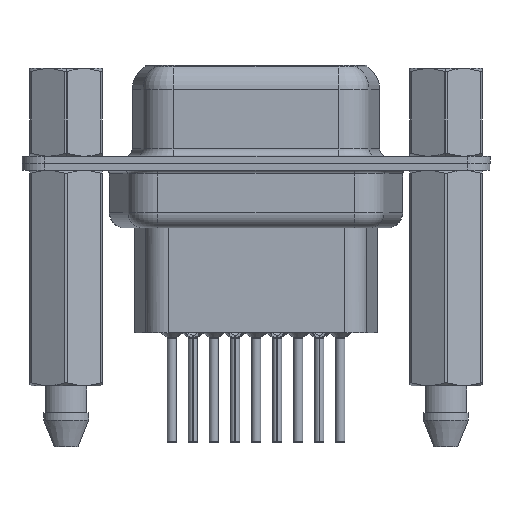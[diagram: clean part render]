
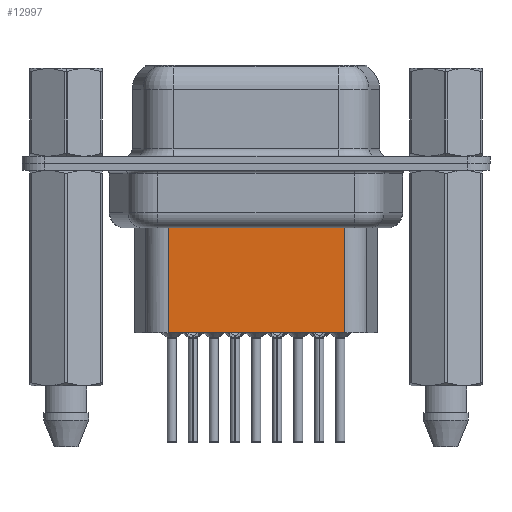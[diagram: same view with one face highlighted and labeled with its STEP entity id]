
A CAD part, front view. The second image highlights one B-rep face of the part: STEP entity #12997.
In plain terms, the highlighted planar face has unit normal (0, -1, 0).
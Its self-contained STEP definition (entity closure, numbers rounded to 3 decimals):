
#63 = DIRECTION ( 'NONE',  ( 1., 0., 0. ) ) ;
#1953 = EDGE_CURVE ( 'NONE', #2417, #6417, #15155, .T. ) ;
#2001 = CARTESIAN_POINT ( 'NONE',  ( 6.706, -3.5, -4.097 ) ) ;
#2026 = ORIENTED_EDGE ( 'NONE', *, *, #19617, .T. ) ;
#2080 = CARTESIAN_POINT ( 'NONE',  ( 18.294, -3.5, -4.097 ) ) ;
#2417 = VERTEX_POINT ( 'NONE', #2001 ) ;
#4248 = FACE_OUTER_BOUND ( 'NONE', #6671, .T. ) ;
#4279 = CARTESIAN_POINT ( 'NONE',  ( 6.706, -3.5, -3.1 ) ) ;
#5543 = VERTEX_POINT ( 'NONE', #8974 ) ;
#6417 = VERTEX_POINT ( 'NONE', #11678 ) ;
#6671 = EDGE_LOOP ( 'NONE', ( #20335, #2026, #26704, #19144 ) ) ;
#6900 = CARTESIAN_POINT ( 'NONE',  ( 18.294, -3.5, -3.1 ) ) ;
#7038 = DIRECTION ( 'NONE',  ( 0., 0., -1. ) ) ;
#7394 = DIRECTION ( 'NONE',  ( -1., 0., 0. ) ) ;
#8974 = CARTESIAN_POINT ( 'NONE',  ( 18.294, -3.5, -11.15 ) ) ;
#9380 = VERTEX_POINT ( 'NONE', #2080 ) ;
#10686 = CARTESIAN_POINT ( 'NONE',  ( 6.706, -3.5, -3.1 ) ) ;
#10730 = EDGE_CURVE ( 'NONE', #9380, #5543, #22218, .T. ) ;
#10855 = DIRECTION ( 'NONE',  ( 0., 0., -1. ) ) ;
#11678 = CARTESIAN_POINT ( 'NONE',  ( 6.706, -3.5, -11.15 ) ) ;
#12785 = DIRECTION ( 'NONE',  ( 0., -1., 0. ) ) ;
#12997 = ADVANCED_FACE ( 'NONE', ( #4248 ), #15269, .T. ) ;
#13716 = CARTESIAN_POINT ( 'NONE',  ( 6.706, -3.5, -11.15 ) ) ;
#14919 = VECTOR ( 'NONE', #26959, 1000. ) ;
#15155 = LINE ( 'NONE', #4279, #26448 ) ;
#15269 = PLANE ( 'NONE',  #24943 ) ;
#16325 = VECTOR ( 'NONE', #7394, 1000. ) ;
#19082 = VECTOR ( 'NONE', #7038, 1000. ) ;
#19144 = ORIENTED_EDGE ( 'NONE', *, *, #23351, .F. ) ;
#19617 = EDGE_CURVE ( 'NONE', #9380, #2417, #22495, .T. ) ;
#20335 = ORIENTED_EDGE ( 'NONE', *, *, #10730, .F. ) ;
#21008 = LINE ( 'NONE', #13716, #16325 ) ;
#22208 = CARTESIAN_POINT ( 'NONE',  ( 6.459, -3.5, -4.097 ) ) ;
#22218 = LINE ( 'NONE', #6900, #19082 ) ;
#22495 = LINE ( 'NONE', #22208, #14919 ) ;
#23351 = EDGE_CURVE ( 'NONE', #5543, #6417, #21008, .T. ) ;
#24943 = AXIS2_PLACEMENT_3D ( 'NONE', #10686, #12785, #63 ) ;
#26448 = VECTOR ( 'NONE', #10855, 1000. ) ;
#26704 = ORIENTED_EDGE ( 'NONE', *, *, #1953, .T. ) ;
#26959 = DIRECTION ( 'NONE',  ( -1., 0., 0. ) ) ;
